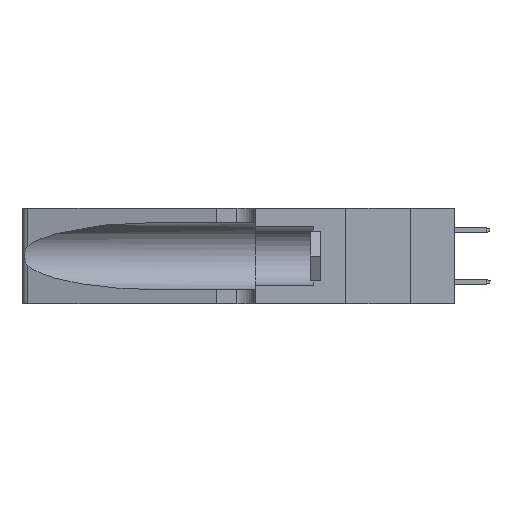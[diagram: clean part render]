
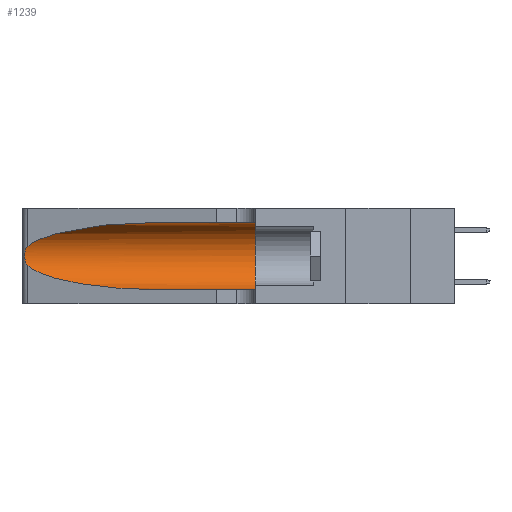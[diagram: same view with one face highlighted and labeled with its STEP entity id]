
A CAD part, left-side view. The second image highlights one B-rep face of the part: STEP entity #1239.
In plain terms, the highlighted cylindrical face has radius 3.308 mm (diameter 6.617 mm), a partial arc.
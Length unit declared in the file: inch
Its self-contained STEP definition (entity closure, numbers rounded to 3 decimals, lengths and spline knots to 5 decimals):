
#304 = DIRECTION ( 'NONE',  ( 0., 0., -1. ) ) ;
#361 = CARTESIAN_POINT ( 'NONE',  ( 0.1305, 1.61858, 0.05475 ) ) ;
#772 = CARTESIAN_POINT ( 'NONE',  ( 0.25856, 1.23593, 0.16098 ) ) ;
#893 = CARTESIAN_POINT ( 'NONE',  ( 0.25555, 1.22994, 0.2215 ) ) ;
#1239 = ADVANCED_FACE ( 'NONE', ( #11541 ), #11165, .F. ) ;
#1611 = AXIS2_PLACEMENT_3D ( 'NONE', #20629, #11408, #304 ) ;
#2865 = CARTESIAN_POINT ( 'NONE',  ( 0.1305, 0.35, 0.31525 ) ) ;
#3302 =( BOUNDED_CURVE ( )  B_SPLINE_CURVE ( 3, ( #5553, #23987, #3691, #18729 ),
 .UNSPECIFIED., .F., .T. ) 
 B_SPLINE_CURVE_WITH_KNOTS ( ( 4, 4 ),
 ( 3.44316, 4.71239 ),
 .UNSPECIFIED. ) 
 CURVE ( )  GEOMETRIC_REPRESENTATION_ITEM ( )  RATIONAL_B_SPLINE_CURVE ( ( 1., 0.87, 0.87, 1. ) ) 
 REPRESENTATION_ITEM ( '' )  );
#3691 = CARTESIAN_POINT ( 'NONE',  ( 0.18966, 0.96281, 0.05475 ) ) ;
#4295 = VERTEX_POINT ( 'NONE', #10763 ) ;
#4459 = CARTESIAN_POINT ( 'NONE',  ( 0.25854, 1.2359, 0.20912 ) ) ;
#4701 = CARTESIAN_POINT ( 'NONE',  ( 0.26018, 1.23835, 0.19895 ) ) ;
#5275 = ORIENTED_EDGE ( 'NONE', *, *, #13820, .T. ) ;
#5553 = CARTESIAN_POINT ( 'NONE',  ( 0.25487, 1.22718, 0.14631 ) ) ;
#5797 = DIRECTION ( 'NONE',  ( 0., 0., 1. ) ) ;
#5904 = DIRECTION ( 'NONE',  ( 0., -1., 0. ) ) ;
#6278 = VERTEX_POINT ( 'NONE', #16794 ) ;
#6520 = EDGE_CURVE ( 'NONE', #10147, #6832, #21554, .T. ) ;
#6663 = CARTESIAN_POINT ( 'NONE',  ( 0.25789, 1.23486, 0.15765 ) ) ;
#6832 = VERTEX_POINT ( 'NONE', #22499 ) ;
#7414 = ORIENTED_EDGE ( 'NONE', *, *, #9941, .T. ) ;
#7563 = CARTESIAN_POINT ( 'NONE',  ( 0.18966, 0.96281, 0.31525 ) ) ;
#7714 = DIRECTION ( 'NONE',  ( 0., -1., 0. ) ) ;
#8290 = CARTESIAN_POINT ( 'NONE',  ( 0.25487, 1.22718, 0.14631 ) ) ;
#9118 = B_SPLINE_CURVE_WITH_KNOTS ( 'NONE', 3,
 ( #14098, #893, #13850, #21603, #4459, #4701, #12226, #11982, #19724, #772, #6663, #14219, #10141, #8290 ),
 .UNSPECIFIED., .F., .F.,
 ( 4, 2, 2, 2, 2, 2, 4 ),
 ( 0., 0.00027, 0.00053, 0.00107, 0.0016, 0.00187, 0.00214 ),
 .UNSPECIFIED. ) ;
#9573 = LINE ( 'NONE', #13251, #10351 ) ;
#9941 = EDGE_CURVE ( 'NONE', #15633, #6278, #9118, .T. ) ;
#10141 = CARTESIAN_POINT ( 'NONE',  ( 0.25555, 1.22993, 0.14849 ) ) ;
#10147 = VERTEX_POINT ( 'NONE', #2865 ) ;
#10351 = VECTOR ( 'NONE', #7714, 39.37008 ) ;
#10763 = CARTESIAN_POINT ( 'NONE',  ( 0.1305, 0.72297, 0.31525 ) ) ;
#10938 = AXIS2_PLACEMENT_3D ( 'NONE', #11482, #22906, #5797 ) ;
#11165 = CYLINDRICAL_SURFACE ( 'NONE', #1611, 0.13025 ) ;
#11351 = EDGE_CURVE ( 'NONE', #14138, #6832, #19323, .T. ) ;
#11390 = ORIENTED_EDGE ( 'NONE', *, *, #20408, .F. ) ;
#11408 = DIRECTION ( 'NONE',  ( 0., -1., 0. ) ) ;
#11482 = CARTESIAN_POINT ( 'NONE',  ( 0.1305, 0.35, 0.185 ) ) ;
#11541 = FACE_OUTER_BOUND ( 'NONE', #19811, .T. ) ;
#11729 = EDGE_CURVE ( 'NONE', #4295, #15633, #23379, .T. ) ;
#11982 = CARTESIAN_POINT ( 'NONE',  ( 0.26075, 1.23896, 0.178 ) ) ;
#12226 = CARTESIAN_POINT ( 'NONE',  ( 0.26075, 1.23896, 0.19203 ) ) ;
#13251 = CARTESIAN_POINT ( 'NONE',  ( 0.1305, 1.61858, 0.31525 ) ) ;
#13820 = EDGE_CURVE ( 'NONE', #6278, #14138, #3302, .T. ) ;
#13850 = CARTESIAN_POINT ( 'NONE',  ( 0.25639, 1.23184, 0.21858 ) ) ;
#14081 = ORIENTED_EDGE ( 'NONE', *, *, #11729, .T. ) ;
#14098 = CARTESIAN_POINT ( 'NONE',  ( 0.25487, 1.22718, 0.22369 ) ) ;
#14138 = VERTEX_POINT ( 'NONE', #17545 ) ;
#14219 = CARTESIAN_POINT ( 'NONE',  ( 0.25639, 1.23186, 0.15144 ) ) ;
#15330 = CARTESIAN_POINT ( 'NONE',  ( 0.1305, 0.72297, 0.31525 ) ) ;
#15633 = VERTEX_POINT ( 'NONE', #21377 ) ;
#16794 = CARTESIAN_POINT ( 'NONE',  ( 0.25487, 1.22718, 0.14631 ) ) ;
#17351 = VECTOR ( 'NONE', #5904, 39.37008 ) ;
#17545 = CARTESIAN_POINT ( 'NONE',  ( 0.1305, 0.72297, 0.05475 ) ) ;
#18729 = CARTESIAN_POINT ( 'NONE',  ( 0.1305, 0.72297, 0.05475 ) ) ;
#19323 = LINE ( 'NONE', #361, #17351 ) ;
#19576 = ORIENTED_EDGE ( 'NONE', *, *, #6520, .F. ) ;
#19724 = CARTESIAN_POINT ( 'NONE',  ( 0.26017, 1.23833, 0.17102 ) ) ;
#19811 = EDGE_LOOP ( 'NONE', ( #14081, #7414, #5275, #21699, #19576, #11390 ) ) ;
#20408 = EDGE_CURVE ( 'NONE', #4295, #10147, #9573, .T. ) ;
#20629 = CARTESIAN_POINT ( 'NONE',  ( 0.1305, 1.61858, 0.185 ) ) ;
#21377 = CARTESIAN_POINT ( 'NONE',  ( 0.25487, 1.22718, 0.22369 ) ) ;
#21554 = CIRCLE ( 'NONE', #10938, 0.13025 ) ;
#21603 = CARTESIAN_POINT ( 'NONE',  ( 0.25787, 1.23484, 0.2124 ) ) ;
#21699 = ORIENTED_EDGE ( 'NONE', *, *, #11351, .T. ) ;
#22499 = CARTESIAN_POINT ( 'NONE',  ( 0.1305, 0.35, 0.05475 ) ) ;
#22701 = CARTESIAN_POINT ( 'NONE',  ( 0.2373, 1.15595, 0.28018 ) ) ;
#22828 = CARTESIAN_POINT ( 'NONE',  ( 0.25487, 1.22718, 0.22369 ) ) ;
#22906 = DIRECTION ( 'NONE',  ( 0., 1., 0. ) ) ;
#23379 =( BOUNDED_CURVE ( )  B_SPLINE_CURVE ( 3, ( #15330, #7563, #22701, #22828 ),
 .UNSPECIFIED., .F., .T. ) 
 B_SPLINE_CURVE_WITH_KNOTS ( ( 4, 4 ),
 ( 1.5708, 2.84003 ),
 .UNSPECIFIED. ) 
 CURVE ( )  GEOMETRIC_REPRESENTATION_ITEM ( )  RATIONAL_B_SPLINE_CURVE ( ( 1., 0.87, 0.87, 1. ) ) 
 REPRESENTATION_ITEM ( '' )  );
#23987 = CARTESIAN_POINT ( 'NONE',  ( 0.2373, 1.15595, 0.08982 ) ) ;
